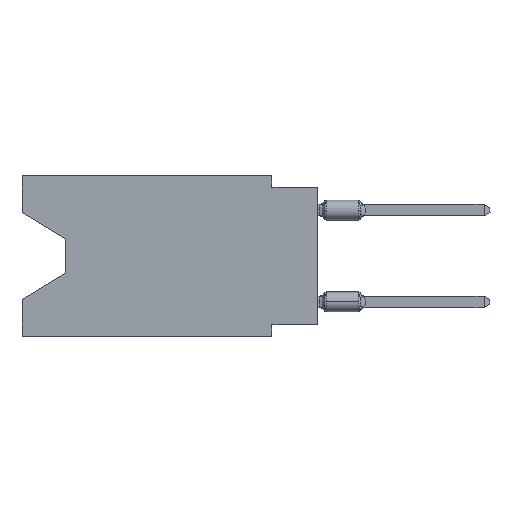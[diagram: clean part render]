
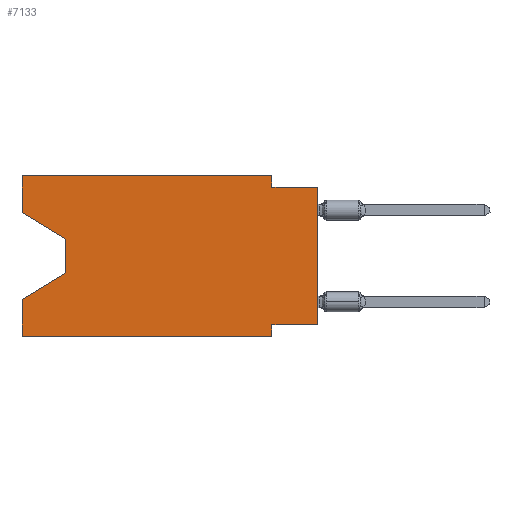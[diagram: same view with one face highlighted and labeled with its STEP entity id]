
A CAD part, left-side view. The second image highlights one B-rep face of the part: STEP entity #7133.
In plain terms, the highlighted planar face has unit normal (-1, 0, 0).
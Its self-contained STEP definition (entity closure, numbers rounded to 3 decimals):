
#66 = VERTEX_POINT ( 'NONE', #2498 ) ;
#146 = VECTOR ( 'NONE', #12659, 1000. ) ;
#338 = CARTESIAN_POINT ( 'NONE',  ( 0., 2.54, -8.255 ) ) ;
#474 = VECTOR ( 'NONE', #12850, 1000. ) ;
#513 = EDGE_CURVE ( 'NONE', #5073, #6228, #12951, .T. ) ;
#725 = DIRECTION ( 'NONE',  ( 1., 0., 0. ) ) ;
#1045 = LINE ( 'NONE', #12572, #5910 ) ;
#1182 = CARTESIAN_POINT ( 'NONE',  ( 0., 16.383, -8.89 ) ) ;
#1475 = EDGE_LOOP ( 'NONE', ( #7618, #11159, #11088, #10179, #10893, #8197, #4208, #9923, #3941, #3936, #11014, #9004 ) ) ;
#1494 = VECTOR ( 'NONE', #13131, 1000. ) ;
#1553 = EDGE_CURVE ( 'NONE', #4949, #2643, #11961, .T. ) ;
#1744 = CARTESIAN_POINT ( 'NONE',  ( 0., 16.383, -2.038 ) ) ;
#1797 = VECTOR ( 'NONE', #11257, 1000. ) ;
#2006 = LINE ( 'NONE', #10384, #9114 ) ;
#2191 = CARTESIAN_POINT ( 'NONE',  ( 0., 2.54, 0. ) ) ;
#2498 = CARTESIAN_POINT ( 'NONE',  ( 0., 0., -8.255 ) ) ;
#2538 = DIRECTION ( 'NONE',  ( 0., 0.855, -0.519 ) ) ;
#2643 = VERTEX_POINT ( 'NONE', #13325 ) ;
#2910 = EDGE_CURVE ( 'NONE', #5945, #5203, #12913, .T. ) ;
#2966 = LINE ( 'NONE', #3037, #146 ) ;
#3003 = DIRECTION ( 'NONE',  ( 0., 0., -1. ) ) ;
#3037 = CARTESIAN_POINT ( 'NONE',  ( 0., 16.383, -8.89 ) ) ;
#3704 = CARTESIAN_POINT ( 'NONE',  ( 0., 13.97, -3.505 ) ) ;
#3936 = ORIENTED_EDGE ( 'NONE', *, *, #11025, .F. ) ;
#3941 = ORIENTED_EDGE ( 'NONE', *, *, #5263, .F. ) ;
#4068 = EDGE_CURVE ( 'NONE', #5203, #7721, #8356, .T. ) ;
#4208 = ORIENTED_EDGE ( 'NONE', *, *, #5350, .F. ) ;
#4449 = CARTESIAN_POINT ( 'NONE',  ( 0., 16.383, 0. ) ) ;
#4450 = EDGE_CURVE ( 'NONE', #4949, #6228, #2966, .T. ) ;
#4480 = CARTESIAN_POINT ( 'NONE',  ( 0., 16.383, 0. ) ) ;
#4511 = LINE ( 'NONE', #8670, #474 ) ;
#4719 = CARTESIAN_POINT ( 'NONE',  ( 0., 16.383, 0. ) ) ;
#4879 = DIRECTION ( 'NONE',  ( 0., 0., -1. ) ) ;
#4949 = VERTEX_POINT ( 'NONE', #1182 ) ;
#5073 = VERTEX_POINT ( 'NONE', #338 ) ;
#5097 = EDGE_CURVE ( 'NONE', #5945, #8199, #4511, .T. ) ;
#5105 = LINE ( 'NONE', #9262, #10948 ) ;
#5203 = VERTEX_POINT ( 'NONE', #13121 ) ;
#5263 = EDGE_CURVE ( 'NONE', #11930, #13214, #8121, .T. ) ;
#5350 = EDGE_CURVE ( 'NONE', #66, #5073, #5105, .T. ) ;
#5389 = VECTOR ( 'NONE', #7756, 1000. ) ;
#5593 = CARTESIAN_POINT ( 'NONE',  ( 0., 2.54, -0.635 ) ) ;
#5898 = VECTOR ( 'NONE', #6332, 1000. ) ;
#5910 = VECTOR ( 'NONE', #9434, 1000. ) ;
#5945 = VERTEX_POINT ( 'NONE', #1744 ) ;
#6094 = VECTOR ( 'NONE', #8540, 1000. ) ;
#6228 = VERTEX_POINT ( 'NONE', #6504 ) ;
#6332 = DIRECTION ( 'NONE',  ( 0., -1., 0. ) ) ;
#6396 = EDGE_CURVE ( 'NONE', #8199, #13094, #10165, .T. ) ;
#6504 = CARTESIAN_POINT ( 'NONE',  ( 0., 2.54, -8.89 ) ) ;
#7133 = ADVANCED_FACE ( 'NONE', ( #7957 ), #9931, .F. ) ;
#7616 = VECTOR ( 'NONE', #3003, 1000. ) ;
#7618 = ORIENTED_EDGE ( 'NONE', *, *, #5097, .T. ) ;
#7721 = VERTEX_POINT ( 'NONE', #2191 ) ;
#7756 = DIRECTION ( 'NONE',  ( 0., 0., -1. ) ) ;
#7957 = FACE_OUTER_BOUND ( 'NONE', #1475, .T. ) ;
#8121 = LINE ( 'NONE', #12281, #1797 ) ;
#8188 = EDGE_CURVE ( 'NONE', #13094, #2643, #8676, .T. ) ;
#8197 = ORIENTED_EDGE ( 'NONE', *, *, #513, .F. ) ;
#8199 = VERTEX_POINT ( 'NONE', #3704 ) ;
#8225 = VECTOR ( 'NONE', #2538, 1000. ) ;
#8356 = LINE ( 'NONE', #4480, #5898 ) ;
#8540 = DIRECTION ( 'NONE',  ( 0., 0., 1. ) ) ;
#8670 = CARTESIAN_POINT ( 'NONE',  ( 0., 16.383, -2.038 ) ) ;
#8676 = LINE ( 'NONE', #12854, #8225 ) ;
#9004 = ORIENTED_EDGE ( 'NONE', *, *, #2910, .F. ) ;
#9114 = VECTOR ( 'NONE', #9224, 1000. ) ;
#9224 = DIRECTION ( 'NONE',  ( 0., 0., -1. ) ) ;
#9262 = CARTESIAN_POINT ( 'NONE',  ( 0., 0., -8.255 ) ) ;
#9434 = DIRECTION ( 'NONE',  ( 0., 0., 1. ) ) ;
#9677 = CARTESIAN_POINT ( 'NONE',  ( 0., 2.54, -8.89 ) ) ;
#9923 = ORIENTED_EDGE ( 'NONE', *, *, #12918, .T. ) ;
#9931 = PLANE ( 'NONE',  #10345 ) ;
#10076 = CARTESIAN_POINT ( 'NONE',  ( 0., 16.383, 0. ) ) ;
#10165 = LINE ( 'NONE', #10238, #7616 ) ;
#10179 = ORIENTED_EDGE ( 'NONE', *, *, #1553, .F. ) ;
#10238 = CARTESIAN_POINT ( 'NONE',  ( 0., 13.97, -3.505 ) ) ;
#10345 = AXIS2_PLACEMENT_3D ( 'NONE', #10076, #725, #4879 ) ;
#10384 = CARTESIAN_POINT ( 'NONE',  ( 0., 2.54, 0. ) ) ;
#10680 = CARTESIAN_POINT ( 'NONE',  ( 0., 13.97, -5.385 ) ) ;
#10893 = ORIENTED_EDGE ( 'NONE', *, *, #4450, .T. ) ;
#10948 = VECTOR ( 'NONE', #11667, 1000. ) ;
#11014 = ORIENTED_EDGE ( 'NONE', *, *, #4068, .F. ) ;
#11025 = EDGE_CURVE ( 'NONE', #7721, #11930, #2006, .T. ) ;
#11088 = ORIENTED_EDGE ( 'NONE', *, *, #8188, .T. ) ;
#11159 = ORIENTED_EDGE ( 'NONE', *, *, #6396, .T. ) ;
#11257 = DIRECTION ( 'NONE',  ( 0., -1., 0. ) ) ;
#11667 = DIRECTION ( 'NONE',  ( 0., 1., 0. ) ) ;
#11930 = VERTEX_POINT ( 'NONE', #5593 ) ;
#11961 = LINE ( 'NONE', #4719, #1494 ) ;
#12278 = CARTESIAN_POINT ( 'NONE',  ( 0., 0., -0.635 ) ) ;
#12281 = CARTESIAN_POINT ( 'NONE',  ( 0., 0., -0.635 ) ) ;
#12572 = CARTESIAN_POINT ( 'NONE',  ( 0., 0., 0. ) ) ;
#12659 = DIRECTION ( 'NONE',  ( 0., -1., 0. ) ) ;
#12850 = DIRECTION ( 'NONE',  ( 0., -0.855, -0.519 ) ) ;
#12854 = CARTESIAN_POINT ( 'NONE',  ( 0., 13.97, -5.385 ) ) ;
#12913 = LINE ( 'NONE', #4449, #6094 ) ;
#12918 = EDGE_CURVE ( 'NONE', #66, #13214, #1045, .T. ) ;
#12951 = LINE ( 'NONE', #9677, #5389 ) ;
#13094 = VERTEX_POINT ( 'NONE', #10680 ) ;
#13121 = CARTESIAN_POINT ( 'NONE',  ( 0., 16.383, 0. ) ) ;
#13131 = DIRECTION ( 'NONE',  ( 0., 0., 1. ) ) ;
#13214 = VERTEX_POINT ( 'NONE', #12278 ) ;
#13325 = CARTESIAN_POINT ( 'NONE',  ( 0., 16.383, -6.852 ) ) ;
